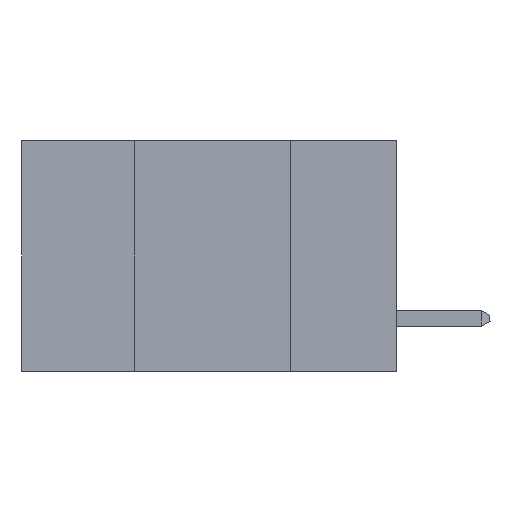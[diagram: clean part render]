
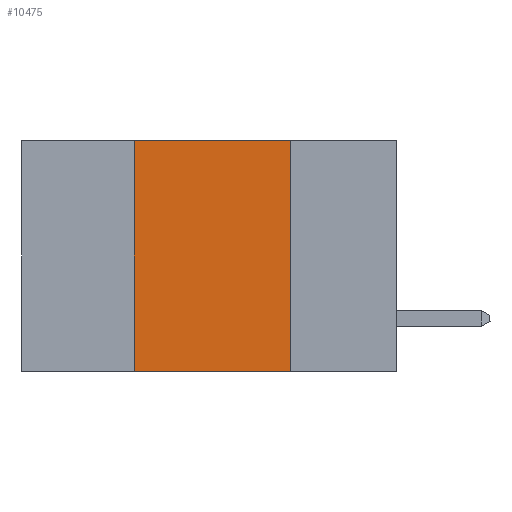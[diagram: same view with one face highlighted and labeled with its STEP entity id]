
A CAD part, left-side view. The second image highlights one B-rep face of the part: STEP entity #10475.
In plain terms, the highlighted planar face has unit normal (-1, 0, 0).
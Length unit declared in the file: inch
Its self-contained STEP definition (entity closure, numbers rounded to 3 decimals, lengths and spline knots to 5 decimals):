
#45 = VECTOR ( 'NONE', #11013, 39.37008 ) ;
#191 = VERTEX_POINT ( 'NONE', #2674 ) ;
#456 = CARTESIAN_POINT ( 'NONE',  ( 0., 0.42, 0. ) ) ;
#798 = VECTOR ( 'NONE', #4368, 39.37008 ) ;
#990 = DIRECTION ( 'NONE',  ( 0., -1., 0. ) ) ;
#1115 = VERTEX_POINT ( 'NONE', #4699 ) ;
#1176 = DIRECTION ( 'NONE',  ( 1., 0., 0. ) ) ;
#1207 = FACE_OUTER_BOUND ( 'NONE', #2761, .T. ) ;
#1417 = ORIENTED_EDGE ( 'NONE', *, *, #9665, .F. ) ;
#2043 = CARTESIAN_POINT ( 'NONE',  ( 0., 0.6, 0. ) ) ;
#2639 = LINE ( 'NONE', #7998, #798 ) ;
#2674 = CARTESIAN_POINT ( 'NONE',  ( 0., 0.42, -0.37 ) ) ;
#2761 = EDGE_LOOP ( 'NONE', ( #8200, #1417, #10743, #9027 ) ) ;
#3461 = VERTEX_POINT ( 'NONE', #4473 ) ;
#3617 = VERTEX_POINT ( 'NONE', #7266 ) ;
#3712 = CARTESIAN_POINT ( 'NONE',  ( 0., 0.17, 0. ) ) ;
#3768 = LINE ( 'NONE', #6419, #4055 ) ;
#4055 = VECTOR ( 'NONE', #990, 39.37008 ) ;
#4368 = DIRECTION ( 'NONE',  ( 0., -1., 0. ) ) ;
#4451 = AXIS2_PLACEMENT_3D ( 'NONE', #2043, #1176, #4781 ) ;
#4473 = CARTESIAN_POINT ( 'NONE',  ( 0., 0.17, 0. ) ) ;
#4699 = CARTESIAN_POINT ( 'NONE',  ( 0., 0.17, -0.37 ) ) ;
#4781 = DIRECTION ( 'NONE',  ( 0., 0., -1. ) ) ;
#6024 = VECTOR ( 'NONE', #8684, 39.37008 ) ;
#6419 = CARTESIAN_POINT ( 'NONE',  ( 0., 0.6, -0.37 ) ) ;
#6553 = EDGE_CURVE ( 'NONE', #3461, #1115, #8449, .T. ) ;
#7266 = CARTESIAN_POINT ( 'NONE',  ( 0., 0.42, 0. ) ) ;
#7998 = CARTESIAN_POINT ( 'NONE',  ( 0., 0.6, 0. ) ) ;
#8200 = ORIENTED_EDGE ( 'NONE', *, *, #6553, .F. ) ;
#8449 = LINE ( 'NONE', #3712, #45 ) ;
#8684 = DIRECTION ( 'NONE',  ( 0., 0., 1. ) ) ;
#9027 = ORIENTED_EDGE ( 'NONE', *, *, #9246, .T. ) ;
#9246 = EDGE_CURVE ( 'NONE', #191, #1115, #3768, .T. ) ;
#9665 = EDGE_CURVE ( 'NONE', #3617, #3461, #2639, .T. ) ;
#10163 = PLANE ( 'NONE',  #4451 ) ;
#10475 = ADVANCED_FACE ( 'NONE', ( #1207 ), #10163, .F. ) ;
#10633 = EDGE_CURVE ( 'NONE', #191, #3617, #10791, .T. ) ;
#10743 = ORIENTED_EDGE ( 'NONE', *, *, #10633, .F. ) ;
#10791 = LINE ( 'NONE', #456, #6024 ) ;
#11013 = DIRECTION ( 'NONE',  ( 0., 0., -1. ) ) ;
